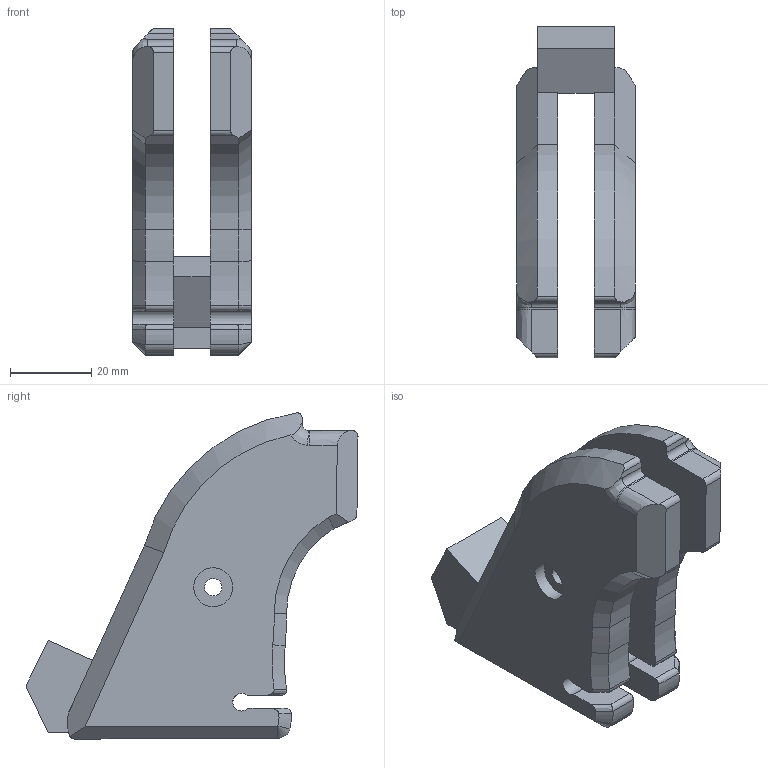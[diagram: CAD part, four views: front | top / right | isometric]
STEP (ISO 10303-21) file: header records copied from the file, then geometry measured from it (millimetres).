
FILE_DESCRIPTION(/* description */ (''),/* implementation_level */ '2;1');
FILE_NAME(/* name */ '7c358137-305f-46a9-9ec2-ab0dc46c822f.stp',/* time_stamp */ '2019-11-26T06:39:27+00:00',/* author */ (''),/* organization */ (''),/* preprocessor_version */ 'ST-DEVELOPER v18',/* originating_system */ 'Autodesk Translation Framework v8.12.0.6',/* authorisation */ '');
FILE_SCHEMA (('AUTOMOTIVE_DESIGN { 1 0 10303 214 3 1 1 }'));
Length unit declared in the file: inch
Products named in the file (1): Heritage Rough Rider - Buffer Tube + Grip Adapter
Bounding box: 29.21 x 81.84 x 80.41 mm (x, y, z)
Volume: 68691.2 mm3; surface area: 19719.9 mm2
Topology: 1 solids, 1 shells, 97 faces, 273 edges, 175 vertices
Faces by surface type: plane 41, cylinder 33, cone 13, bspline 10
Full cylindrical faces by diameter (mm): 4.305 x2, 9.604 x1
Entity records: 3756 total; most frequent: CARTESIAN_POINT 1269, ORIENTED_EDGE 546, DIRECTION 476, EDGE_CURVE 273, VERTEX_POINT 175, AXIS2_PLACEMENT_3D 165, LINE 146, VECTOR 146
